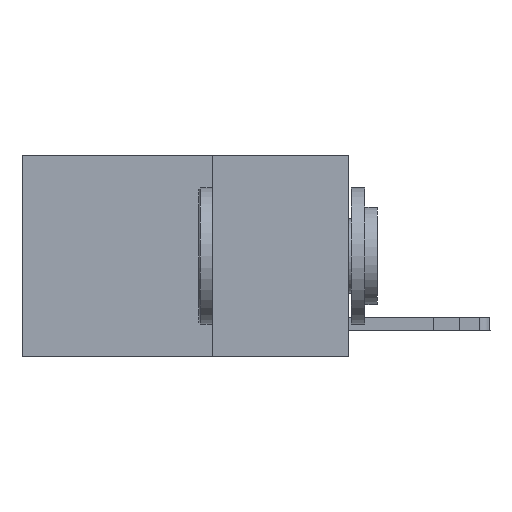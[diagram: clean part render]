
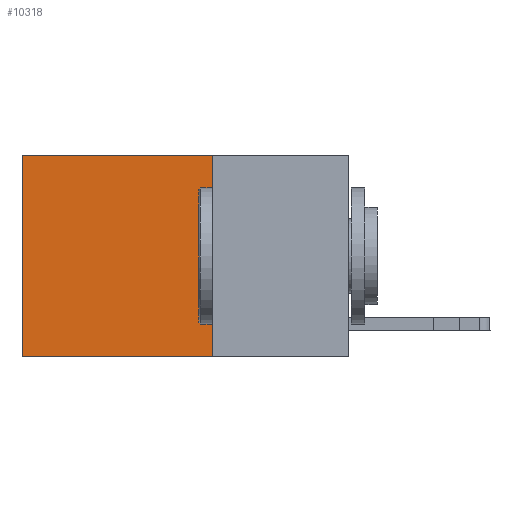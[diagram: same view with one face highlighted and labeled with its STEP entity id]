
A CAD part, left-side view. The second image highlights one B-rep face of the part: STEP entity #10318.
In plain terms, the highlighted planar face has unit normal (-1, 0, 0).
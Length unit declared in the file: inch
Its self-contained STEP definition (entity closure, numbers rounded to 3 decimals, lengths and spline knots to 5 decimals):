
#742 = ORIENTED_EDGE ( 'NONE', *, *, #17681, .F. ) ;
#1123 = CARTESIAN_POINT ( 'NONE',  ( 0.2625, 0.25, 0. ) ) ;
#1273 = VERTEX_POINT ( 'NONE', #10370 ) ;
#1788 = EDGE_CURVE ( 'NONE', #14262, #4209, #15992, .T. ) ;
#1990 = LINE ( 'NONE', #4871, #17783 ) ;
#2127 = DIRECTION ( 'NONE',  ( 0., 1., 0. ) ) ;
#2237 = VERTEX_POINT ( 'NONE', #14563 ) ;
#3061 = ORIENTED_EDGE ( 'NONE', *, *, #1788, .T. ) ;
#3087 = CARTESIAN_POINT ( 'NONE',  ( 0.2625, 0.6, 0. ) ) ;
#3724 = CARTESIAN_POINT ( 'NONE',  ( 0.2625, 0.6, -0.37 ) ) ;
#4209 = VERTEX_POINT ( 'NONE', #3724 ) ;
#4871 = CARTESIAN_POINT ( 'NONE',  ( 0.2625, 0.25, 0. ) ) ;
#5867 = AXIS2_PLACEMENT_3D ( 'NONE', #10746, #8141, #16402 ) ;
#5973 = EDGE_CURVE ( 'NONE', #2237, #14262, #6722, .T. ) ;
#6722 = LINE ( 'NONE', #1123, #8765 ) ;
#7968 = FACE_OUTER_BOUND ( 'NONE', #15917, .T. ) ;
#8141 = DIRECTION ( 'NONE',  ( 1., 0., 0. ) ) ;
#8494 = ORIENTED_EDGE ( 'NONE', *, *, #13729, .F. ) ;
#8765 = VECTOR ( 'NONE', #16536, 39.37008 ) ;
#9249 = CARTESIAN_POINT ( 'NONE',  ( 0.2625, 0.6, 0. ) ) ;
#9694 = ORIENTED_EDGE ( 'NONE', *, *, #5973, .T. ) ;
#10318 = ADVANCED_FACE ( 'NONE', ( #7968 ), #13624, .F. ) ;
#10370 = CARTESIAN_POINT ( 'NONE',  ( 0.2625, 0.25, -0.37 ) ) ;
#10491 = VECTOR ( 'NONE', #2127, 39.37008 ) ;
#10746 = CARTESIAN_POINT ( 'NONE',  ( 0.2625, 0.25, 0. ) ) ;
#13624 = PLANE ( 'NONE',  #5867 ) ;
#13729 = EDGE_CURVE ( 'NONE', #2237, #1273, #1990, .T. ) ;
#14262 = VERTEX_POINT ( 'NONE', #9249 ) ;
#14483 = VECTOR ( 'NONE', #17125, 39.37008 ) ;
#14563 = CARTESIAN_POINT ( 'NONE',  ( 0.2625, 0.25, 0. ) ) ;
#15066 = CARTESIAN_POINT ( 'NONE',  ( 0.2625, 0.25, -0.37 ) ) ;
#15917 = EDGE_LOOP ( 'NONE', ( #3061, #742, #8494, #9694 ) ) ;
#15992 = LINE ( 'NONE', #3087, #14483 ) ;
#16402 = DIRECTION ( 'NONE',  ( 0., 0., -1. ) ) ;
#16454 = LINE ( 'NONE', #15066, #10491 ) ;
#16536 = DIRECTION ( 'NONE',  ( 0., 1., 0. ) ) ;
#17125 = DIRECTION ( 'NONE',  ( 0., 0., -1. ) ) ;
#17681 = EDGE_CURVE ( 'NONE', #1273, #4209, #16454, .T. ) ;
#17783 = VECTOR ( 'NONE', #17990, 39.37008 ) ;
#17990 = DIRECTION ( 'NONE',  ( 0., 0., -1. ) ) ;
